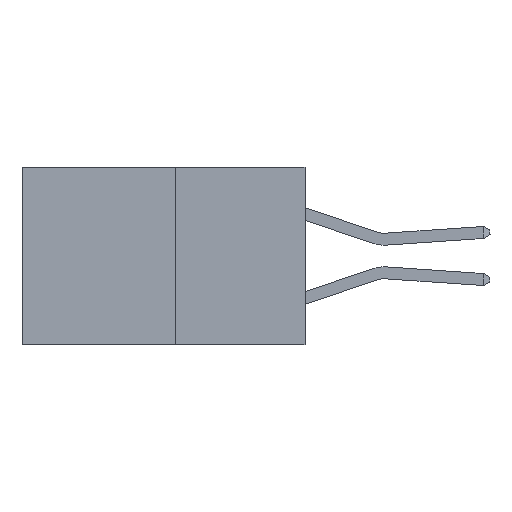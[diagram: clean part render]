
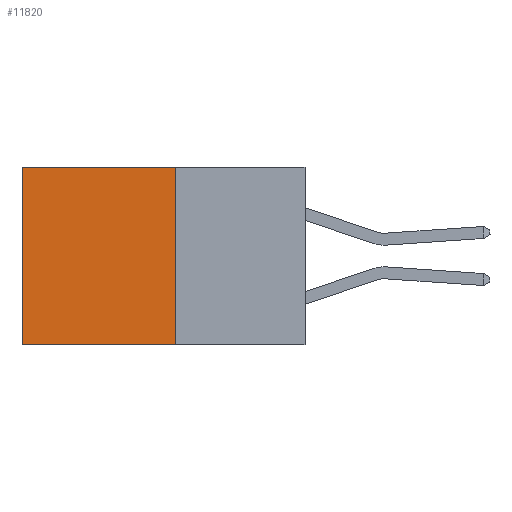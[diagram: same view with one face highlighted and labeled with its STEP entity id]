
A CAD part, left-side view. The second image highlights one B-rep face of the part: STEP entity #11820.
In plain terms, the highlighted planar face has unit normal (-1, 0, 0).
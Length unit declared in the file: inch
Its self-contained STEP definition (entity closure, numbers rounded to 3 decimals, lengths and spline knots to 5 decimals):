
#484 = DIRECTION ( 'NONE',  ( 1., 0., 0. ) ) ;
#947 = ORIENTED_EDGE ( 'NONE', *, *, #1529, .T. ) ;
#1529 = EDGE_CURVE ( 'NONE', #11145, #9569, #8284, .T. ) ;
#1566 = ORIENTED_EDGE ( 'NONE', *, *, #11607, .F. ) ;
#1673 = ORIENTED_EDGE ( 'NONE', *, *, #4682, .F. ) ;
#1861 = CARTESIAN_POINT ( 'NONE',  ( 0.277, 0.59, -0.37 ) ) ;
#2659 = CARTESIAN_POINT ( 'NONE',  ( 0.277, 0.27, -0.37 ) ) ;
#2835 = ORIENTED_EDGE ( 'NONE', *, *, #8746, .T. ) ;
#2983 = EDGE_LOOP ( 'NONE', ( #2835, #1673, #1566, #947 ) ) ;
#4682 = EDGE_CURVE ( 'NONE', #7908, #5000, #12034, .T. ) ;
#5000 = VERTEX_POINT ( 'NONE', #1861 ) ;
#5137 = CARTESIAN_POINT ( 'NONE',  ( 0.277, 0.59, 0. ) ) ;
#5345 = VECTOR ( 'NONE', #14227, 39.37008 ) ;
#5995 = DIRECTION ( 'NONE',  ( 0., 1., 0. ) ) ;
#6020 = CARTESIAN_POINT ( 'NONE',  ( 0.277, 0.27, -0.37 ) ) ;
#6194 = CARTESIAN_POINT ( 'NONE',  ( 0.277, 0.27, -0.37 ) ) ;
#7245 = VECTOR ( 'NONE', #10317, 39.37008 ) ;
#7331 = LINE ( 'NONE', #14090, #10678 ) ;
#7388 = DIRECTION ( 'NONE',  ( 0., 0., -1. ) ) ;
#7908 = VERTEX_POINT ( 'NONE', #6194 ) ;
#8127 = FACE_OUTER_BOUND ( 'NONE', #2983, .T. ) ;
#8284 = LINE ( 'NONE', #14173, #5345 ) ;
#8374 = CARTESIAN_POINT ( 'NONE',  ( 0.277, 0.27, -0.37 ) ) ;
#8418 = DIRECTION ( 'NONE',  ( 0., 0., -1. ) ) ;
#8746 = EDGE_CURVE ( 'NONE', #9569, #5000, #7331, .T. ) ;
#9023 = VECTOR ( 'NONE', #5995, 39.37008 ) ;
#9569 = VERTEX_POINT ( 'NONE', #5137 ) ;
#10212 = LINE ( 'NONE', #2659, #7245 ) ;
#10317 = DIRECTION ( 'NONE',  ( 0., 0., -1. ) ) ;
#10678 = VECTOR ( 'NONE', #7388, 39.37008 ) ;
#11145 = VERTEX_POINT ( 'NONE', #14104 ) ;
#11607 = EDGE_CURVE ( 'NONE', #11145, #7908, #10212, .T. ) ;
#11820 = ADVANCED_FACE ( 'NONE', ( #8127 ), #14017, .F. ) ;
#12034 = LINE ( 'NONE', #6020, #9023 ) ;
#12667 = AXIS2_PLACEMENT_3D ( 'NONE', #8374, #484, #8418 ) ;
#14017 = PLANE ( 'NONE',  #12667 ) ;
#14090 = CARTESIAN_POINT ( 'NONE',  ( 0.277, 0.59, -0.37 ) ) ;
#14104 = CARTESIAN_POINT ( 'NONE',  ( 0.277, 0.27, 0. ) ) ;
#14173 = CARTESIAN_POINT ( 'NONE',  ( 0.277, 0.27, 0. ) ) ;
#14227 = DIRECTION ( 'NONE',  ( 0., 1., 0. ) ) ;
